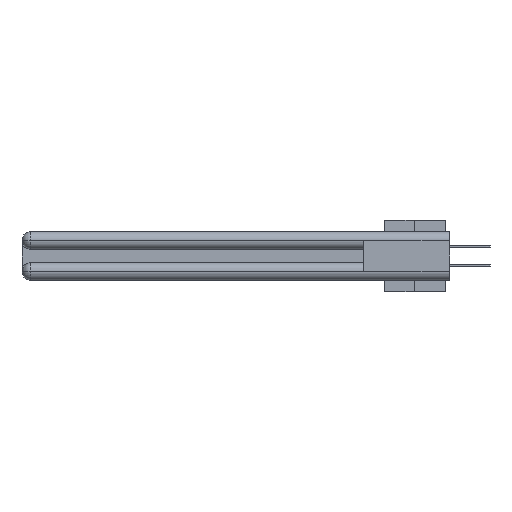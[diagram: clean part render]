
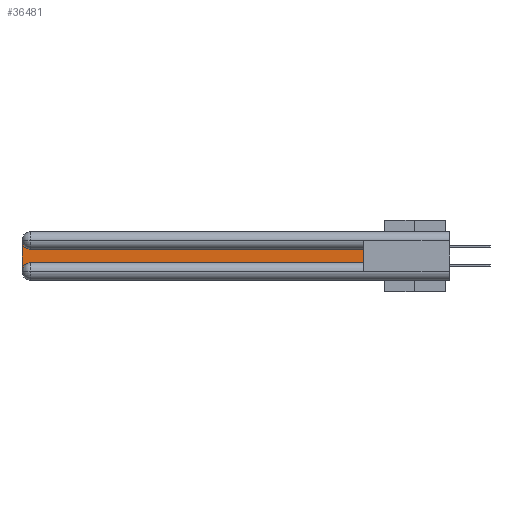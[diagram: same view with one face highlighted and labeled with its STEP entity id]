
A CAD part, left-side view. The second image highlights one B-rep face of the part: STEP entity #36481.
In plain terms, the highlighted planar face has unit normal (-1, 0, 0).
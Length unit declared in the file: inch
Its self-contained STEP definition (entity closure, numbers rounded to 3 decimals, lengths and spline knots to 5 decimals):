
#58 = VECTOR ( 'NONE', #39776, 39.37008 ) ;
#2853 = CARTESIAN_POINT ( 'NONE',  ( 0.075, 0.6, -0.2175 ) ) ;
#7075 = CARTESIAN_POINT ( 'NONE',  ( 0.075, 3., -0.2775 ) ) ;
#7769 = VERTEX_POINT ( 'NONE', #22297 ) ;
#7815 = ORIENTED_EDGE ( 'NONE', *, *, #44288, .T. ) ;
#8201 = LINE ( 'NONE', #40869, #19453 ) ;
#8313 = LINE ( 'NONE', #41269, #24359 ) ;
#9693 = DIRECTION ( 'NONE',  ( 0., 0., -1. ) ) ;
#10767 = DIRECTION ( 'NONE',  ( 1., 0., 0. ) ) ;
#11198 = VERTEX_POINT ( 'NONE', #7075 ) ;
#12328 = DIRECTION ( 'NONE',  ( 0., 0., -1. ) ) ;
#14766 = AXIS2_PLACEMENT_3D ( 'NONE', #19747, #20255, #12328 ) ;
#15148 = PLANE ( 'NONE',  #28851 ) ;
#17623 = VECTOR ( 'NONE', #9693, 39.37008 ) ;
#19380 = LINE ( 'NONE', #21442, #17623 ) ;
#19453 = VECTOR ( 'NONE', #44063, 39.37008 ) ;
#19747 = CARTESIAN_POINT ( 'NONE',  ( 0.075, 2.94, -0.2775 ) ) ;
#20255 = DIRECTION ( 'NONE',  ( 1., 0., 0. ) ) ;
#20696 = ORIENTED_EDGE ( 'NONE', *, *, #33370, .T. ) ;
#21109 = ORIENTED_EDGE ( 'NONE', *, *, #35475, .T. ) ;
#21442 = CARTESIAN_POINT ( 'NONE',  ( 0.075, 3., -0.2175 ) ) ;
#21876 = CARTESIAN_POINT ( 'NONE',  ( 0.075, 2.94, -0.1225 ) ) ;
#22297 = CARTESIAN_POINT ( 'NONE',  ( 0.075, 0.6, -0.1225 ) ) ;
#22891 = VERTEX_POINT ( 'NONE', #21876 ) ;
#22928 = ORIENTED_EDGE ( 'NONE', *, *, #43858, .T. ) ;
#23007 = ORIENTED_EDGE ( 'NONE', *, *, #28506, .T. ) ;
#24197 = CIRCLE ( 'NONE', #14766, 0.06 ) ;
#24359 = VECTOR ( 'NONE', #25872, 39.37008 ) ;
#25684 = EDGE_CURVE ( 'NONE', #39590, #7769, #8201, .T. ) ;
#25872 = DIRECTION ( 'NONE',  ( 0., 1., 0. ) ) ;
#26499 = DIRECTION ( 'NONE',  ( 0., 0., -1. ) ) ;
#26502 = CARTESIAN_POINT ( 'NONE',  ( 0.075, 3., -0.0625 ) ) ;
#26679 = LINE ( 'NONE', #42968, #58 ) ;
#27805 = CIRCLE ( 'NONE', #36405, 0.06 ) ;
#28506 = EDGE_CURVE ( 'NONE', #41621, #11198, #19380, .T. ) ;
#28851 = AXIS2_PLACEMENT_3D ( 'NONE', #30067, #33881, #41680 ) ;
#30067 = CARTESIAN_POINT ( 'NONE',  ( 0.075, 3., -0.1225 ) ) ;
#33370 = EDGE_CURVE ( 'NONE', #39751, #39590, #26679, .T. ) ;
#33647 = CARTESIAN_POINT ( 'NONE',  ( 0.075, 2.94, -0.0625 ) ) ;
#33881 = DIRECTION ( 'NONE',  ( 1., 0., 0. ) ) ;
#34109 = CARTESIAN_POINT ( 'NONE',  ( 0.075, 2.94, -0.2175 ) ) ;
#34329 = FACE_OUTER_BOUND ( 'NONE', #41569, .T. ) ;
#35340 = ORIENTED_EDGE ( 'NONE', *, *, #25684, .T. ) ;
#35475 = EDGE_CURVE ( 'NONE', #7769, #22891, #8313, .T. ) ;
#36405 = AXIS2_PLACEMENT_3D ( 'NONE', #33647, #10767, #26499 ) ;
#36481 = ADVANCED_FACE ( 'NONE', ( #34329 ), #15148, .F. ) ;
#39590 = VERTEX_POINT ( 'NONE', #2853 ) ;
#39751 = VERTEX_POINT ( 'NONE', #34109 ) ;
#39776 = DIRECTION ( 'NONE',  ( 0., -1., 0. ) ) ;
#40869 = CARTESIAN_POINT ( 'NONE',  ( 0.075, 0.6, -0.2175 ) ) ;
#41269 = CARTESIAN_POINT ( 'NONE',  ( 0.075, 0.6, -0.1225 ) ) ;
#41569 = EDGE_LOOP ( 'NONE', ( #21109, #7815, #23007, #22928, #20696, #35340 ) ) ;
#41621 = VERTEX_POINT ( 'NONE', #26502 ) ;
#41680 = DIRECTION ( 'NONE',  ( 0., 0., -1. ) ) ;
#42968 = CARTESIAN_POINT ( 'NONE',  ( 0.075, 0.6, -0.2175 ) ) ;
#43858 = EDGE_CURVE ( 'NONE', #11198, #39751, #24197, .T. ) ;
#44063 = DIRECTION ( 'NONE',  ( 0., 0., 1. ) ) ;
#44288 = EDGE_CURVE ( 'NONE', #22891, #41621, #27805, .T. ) ;
